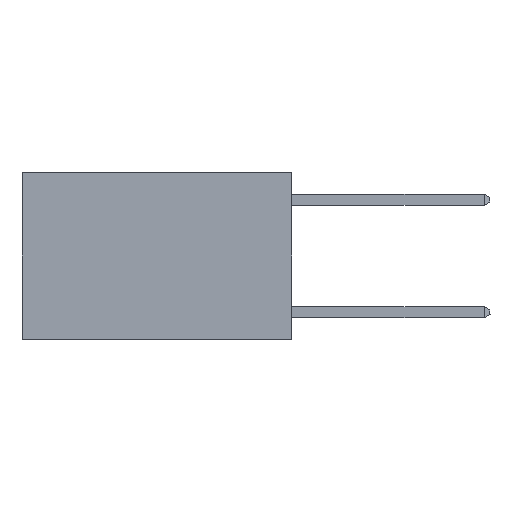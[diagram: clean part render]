
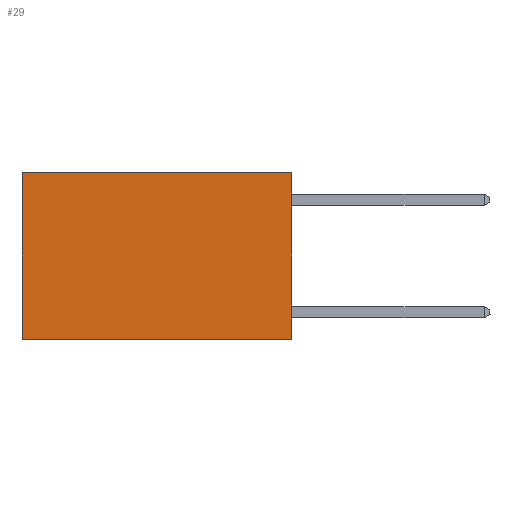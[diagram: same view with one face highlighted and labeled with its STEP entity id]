
A CAD part, left-side view. The second image highlights one B-rep face of the part: STEP entity #29.
In plain terms, the highlighted planar face has unit normal (-1, 0, 0).
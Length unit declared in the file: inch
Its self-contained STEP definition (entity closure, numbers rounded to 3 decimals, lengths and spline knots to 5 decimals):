
#29 = ADVANCED_FACE ( 'NONE', ( #8157 ), #5766, .F. ) ;
#1813 = EDGE_CURVE ( 'NONE', #2699, #11609, #17196, .T. ) ;
#1817 = LINE ( 'NONE', #6250, #12285 ) ;
#2699 = VERTEX_POINT ( 'NONE', #15282 ) ;
#2824 = VECTOR ( 'NONE', #3104, 39.37008 ) ;
#3100 = ORIENTED_EDGE ( 'NONE', *, *, #1813, .T. ) ;
#3104 = DIRECTION ( 'NONE',  ( 0., 0., -1. ) ) ;
#3511 = ORIENTED_EDGE ( 'NONE', *, *, #17197, .F. ) ;
#4560 = ORIENTED_EDGE ( 'NONE', *, *, #12050, .F. ) ;
#4598 = ORIENTED_EDGE ( 'NONE', *, *, #14762, .T. ) ;
#4871 = EDGE_LOOP ( 'NONE', ( #3100, #3511, #4560, #4598 ) ) ;
#5083 = VECTOR ( 'NONE', #8235, 39.37008 ) ;
#5509 = LINE ( 'NONE', #14698, #5083 ) ;
#5766 = PLANE ( 'NONE',  #9773 ) ;
#6197 = VERTEX_POINT ( 'NONE', #9533 ) ;
#6250 = CARTESIAN_POINT ( 'NONE',  ( 0.2625, 0., 0. ) ) ;
#6817 = VECTOR ( 'NONE', #11232, 39.37008 ) ;
#7379 = DIRECTION ( 'NONE',  ( 0., 0., -1. ) ) ;
#7606 = DIRECTION ( 'NONE',  ( 0., 1., 0. ) ) ;
#8157 = FACE_OUTER_BOUND ( 'NONE', #4871, .T. ) ;
#8235 = DIRECTION ( 'NONE',  ( 0., 1., 0. ) ) ;
#8723 = CARTESIAN_POINT ( 'NONE',  ( 0.2625, 0.6, -0.37 ) ) ;
#8858 = CARTESIAN_POINT ( 'NONE',  ( 0.2625, 0., -0.37 ) ) ;
#9533 = CARTESIAN_POINT ( 'NONE',  ( 0.2625, 0., 0. ) ) ;
#9773 = AXIS2_PLACEMENT_3D ( 'NONE', #16488, #13073, #7379 ) ;
#11002 = VERTEX_POINT ( 'NONE', #8858 ) ;
#11219 = CARTESIAN_POINT ( 'NONE',  ( 0.2625, 0., 0. ) ) ;
#11232 = DIRECTION ( 'NONE',  ( 0., 0., -1. ) ) ;
#11609 = VERTEX_POINT ( 'NONE', #8723 ) ;
#12050 = EDGE_CURVE ( 'NONE', #6197, #11002, #17302, .T. ) ;
#12285 = VECTOR ( 'NONE', #7606, 39.37008 ) ;
#12542 = CARTESIAN_POINT ( 'NONE',  ( 0.2625, 0.6, 0. ) ) ;
#13073 = DIRECTION ( 'NONE',  ( 1., 0., 0. ) ) ;
#14698 = CARTESIAN_POINT ( 'NONE',  ( 0.2625, 0., -0.37 ) ) ;
#14762 = EDGE_CURVE ( 'NONE', #6197, #2699, #1817, .T. ) ;
#15282 = CARTESIAN_POINT ( 'NONE',  ( 0.2625, 0.6, 0. ) ) ;
#16488 = CARTESIAN_POINT ( 'NONE',  ( 0.2625, 0., 0. ) ) ;
#17196 = LINE ( 'NONE', #12542, #6817 ) ;
#17197 = EDGE_CURVE ( 'NONE', #11002, #11609, #5509, .T. ) ;
#17302 = LINE ( 'NONE', #11219, #2824 ) ;
